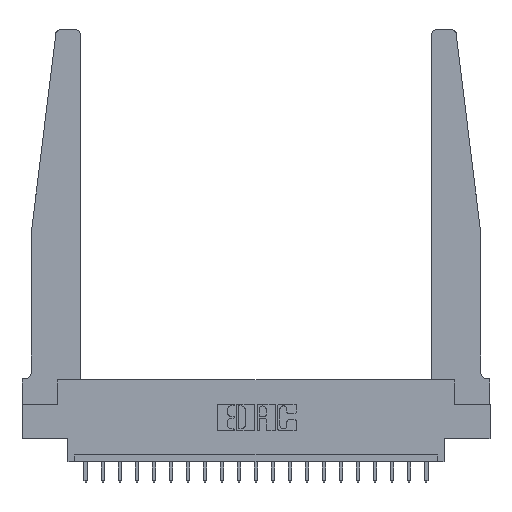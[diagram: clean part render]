
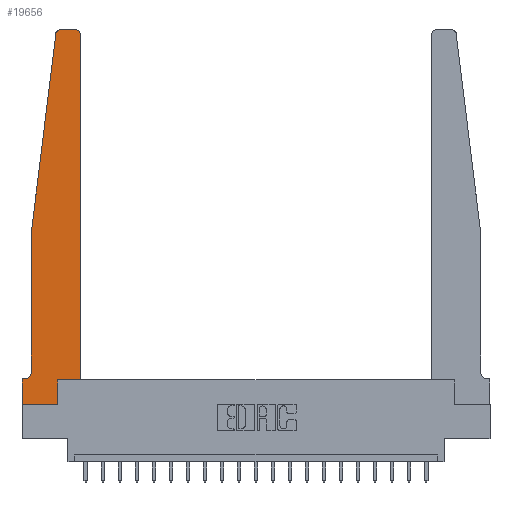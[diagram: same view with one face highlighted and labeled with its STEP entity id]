
A CAD part, top view. The second image highlights one B-rep face of the part: STEP entity #19656.
In plain terms, the highlighted planar face has unit normal (0, 0, 1).
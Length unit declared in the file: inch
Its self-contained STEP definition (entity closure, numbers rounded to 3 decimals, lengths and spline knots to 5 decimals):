
#21 = CARTESIAN_POINT ( 'NONE',  ( 0.065, 0.2375, 0.37 ) ) ;
#108 = VERTEX_POINT ( 'NONE', #7476 ) ;
#614 = LINE ( 'NONE', #13580, #15543 ) ;
#941 = DIRECTION ( 'NONE',  ( 1., 0., 0. ) ) ;
#1406 = EDGE_CURVE ( 'NONE', #4958, #7161, #15280, .T. ) ;
#1750 = CARTESIAN_POINT ( 'NONE',  ( 0.2605, 0.18, 0.37 ) ) ;
#2134 = ORIENTED_EDGE ( 'NONE', *, *, #15273, .T. ) ;
#2272 = ORIENTED_EDGE ( 'NONE', *, *, #1406, .T. ) ;
#2599 = DIRECTION ( 'NONE',  ( 0., 0., -1. ) ) ;
#2817 = ORIENTED_EDGE ( 'NONE', *, *, #3318, .T. ) ;
#3095 = ORIENTED_EDGE ( 'NONE', *, *, #17655, .T. ) ;
#3299 = ORIENTED_EDGE ( 'NONE', *, *, #13566, .T. ) ;
#3318 = EDGE_CURVE ( 'NONE', #15799, #108, #10245, .T. ) ;
#3681 = AXIS2_PLACEMENT_3D ( 'NONE', #21122, #14451, #14241 ) ;
#3939 = DIRECTION ( 'NONE',  ( 0., -1., 0. ) ) ;
#3965 = EDGE_CURVE ( 'NONE', #4890, #17208, #18164, .T. ) ;
#4087 = AXIS2_PLACEMENT_3D ( 'NONE', #6137, #8046, #15952 ) ;
#4551 = ORIENTED_EDGE ( 'NONE', *, *, #17848, .T. ) ;
#4890 = VERTEX_POINT ( 'NONE', #15218 ) ;
#4958 = VERTEX_POINT ( 'NONE', #20593 ) ;
#5138 = VECTOR ( 'NONE', #11738, 39.37008 ) ;
#5883 = CARTESIAN_POINT ( 'NONE',  ( 0.425, 0.18, 0.37 ) ) ;
#5889 = CARTESIAN_POINT ( 'NONE',  ( 0.425, 0.18, 0.37 ) ) ;
#6137 = CARTESIAN_POINT ( 'NONE',  ( 0.27653, 2.72, 0.37 ) ) ;
#6249 = CARTESIAN_POINT ( 'NONE',  ( 0.395, 2.72, 0.37 ) ) ;
#6349 = DIRECTION ( 'NONE',  ( 1., 0., 0. ) ) ;
#6737 = CARTESIAN_POINT ( 'NONE',  ( 0.065, 1.25, 0.37 ) ) ;
#6746 = EDGE_CURVE ( 'NONE', #108, #14042, #17950, .T. ) ;
#6750 = DIRECTION ( 'NONE',  ( -1., 0., 0. ) ) ;
#6759 = CIRCLE ( 'NONE', #9444, 0.05 ) ;
#7161 = VERTEX_POINT ( 'NONE', #1750 ) ;
#7476 = CARTESIAN_POINT ( 'NONE',  ( 0.24675, 2.72367, 0.37 ) ) ;
#7644 = LINE ( 'NONE', #12654, #20447 ) ;
#8046 = DIRECTION ( 'NONE',  ( 0., 0., 1. ) ) ;
#8259 = CARTESIAN_POINT ( 'NONE',  ( 0.25, 2.75, 0.37 ) ) ;
#8447 = VERTEX_POINT ( 'NONE', #5883 ) ;
#8603 = CARTESIAN_POINT ( 'NONE',  ( 0.425, 0.18, 0.37 ) ) ;
#8801 = LINE ( 'NONE', #8603, #10506 ) ;
#8855 = CARTESIAN_POINT ( 'NONE',  ( 0., 0., 0.37 ) ) ;
#9163 = VERTEX_POINT ( 'NONE', #12025 ) ;
#9293 = CARTESIAN_POINT ( 'NONE',  ( 0.065, 1.25, 0.37 ) ) ;
#9444 = AXIS2_PLACEMENT_3D ( 'NONE', #15856, #2599, #20381 ) ;
#9493 = CARTESIAN_POINT ( 'NONE',  ( 0.425, 2.72, 0.37 ) ) ;
#10059 = ORIENTED_EDGE ( 'NONE', *, *, #11629, .T. ) ;
#10174 = LINE ( 'NONE', #8259, #20086 ) ;
#10245 = CIRCLE ( 'NONE', #4087, 0.03 ) ;
#10506 = VECTOR ( 'NONE', #18427, 39.37008 ) ;
#10508 = AXIS2_PLACEMENT_3D ( 'NONE', #6249, #19416, #6349 ) ;
#11250 = PLANE ( 'NONE',  #3681 ) ;
#11629 = EDGE_CURVE ( 'NONE', #19287, #9163, #19748, .T. ) ;
#11723 = ORIENTED_EDGE ( 'NONE', *, *, #12429, .T. ) ;
#11738 = DIRECTION ( 'NONE',  ( -1., 0., 0. ) ) ;
#12025 = CARTESIAN_POINT ( 'NONE',  ( 0.395, 2.75, 0.37 ) ) ;
#12171 = DIRECTION ( 'NONE',  ( 0., -1., 0. ) ) ;
#12221 = EDGE_CURVE ( 'NONE', #9163, #15799, #10174, .T. ) ;
#12429 = EDGE_CURVE ( 'NONE', #14042, #12829, #614, .T. ) ;
#12654 = CARTESIAN_POINT ( 'NONE',  ( 0., 0., 0.37 ) ) ;
#12687 = CARTESIAN_POINT ( 'NONE',  ( 0., 0.1875, 0.37 ) ) ;
#12829 = VERTEX_POINT ( 'NONE', #21 ) ;
#13028 = VECTOR ( 'NONE', #19688, 39.37008 ) ;
#13553 = CARTESIAN_POINT ( 'NONE',  ( 0.065, 0.1875, 0.37 ) ) ;
#13566 = EDGE_CURVE ( 'NONE', #7161, #8447, #18729, .T. ) ;
#13580 = CARTESIAN_POINT ( 'NONE',  ( 0.065, 1.25, 0.37 ) ) ;
#13930 = VECTOR ( 'NONE', #19025, 39.37008 ) ;
#14042 = VERTEX_POINT ( 'NONE', #9293 ) ;
#14105 = EDGE_LOOP ( 'NONE', ( #16963, #2817, #19801, #11723, #20723, #18368, #2134, #3095, #2272, #3299, #4551, #10059 ) ) ;
#14202 = VECTOR ( 'NONE', #12171, 39.37008 ) ;
#14241 = DIRECTION ( 'NONE',  ( 1., 0., 0. ) ) ;
#14451 = DIRECTION ( 'NONE',  ( 0., 0., 1. ) ) ;
#15118 = VERTEX_POINT ( 'NONE', #8855 ) ;
#15218 = CARTESIAN_POINT ( 'NONE',  ( 0.015, 0.1875, 0.37 ) ) ;
#15273 = EDGE_CURVE ( 'NONE', #17208, #15118, #15393, .T. ) ;
#15280 = LINE ( 'NONE', #20218, #13930 ) ;
#15393 = LINE ( 'NONE', #20329, #14202 ) ;
#15543 = VECTOR ( 'NONE', #3939, 39.37008 ) ;
#15799 = VERTEX_POINT ( 'NONE', #20199 ) ;
#15856 = CARTESIAN_POINT ( 'NONE',  ( 0.015, 0.2375, 0.37 ) ) ;
#15952 = DIRECTION ( 'NONE',  ( 1., 0., 0. ) ) ;
#16963 = ORIENTED_EDGE ( 'NONE', *, *, #12221, .T. ) ;
#17208 = VERTEX_POINT ( 'NONE', #12687 ) ;
#17644 = EDGE_CURVE ( 'NONE', #12829, #4890, #6759, .T. ) ;
#17655 = EDGE_CURVE ( 'NONE', #15118, #4958, #7644, .T. ) ;
#17848 = EDGE_CURVE ( 'NONE', #8447, #19287, #8801, .T. ) ;
#17861 = FACE_OUTER_BOUND ( 'NONE', #14105, .T. ) ;
#17950 = LINE ( 'NONE', #6737, #13028 ) ;
#18164 = LINE ( 'NONE', #13553, #5138 ) ;
#18368 = ORIENTED_EDGE ( 'NONE', *, *, #3965, .T. ) ;
#18427 = DIRECTION ( 'NONE',  ( 0., 1., 0. ) ) ;
#18729 = LINE ( 'NONE', #5889, #20654 ) ;
#18879 = DIRECTION ( 'NONE',  ( 1., 0., 0. ) ) ;
#19025 = DIRECTION ( 'NONE',  ( 0., 1., 0. ) ) ;
#19287 = VERTEX_POINT ( 'NONE', #9493 ) ;
#19416 = DIRECTION ( 'NONE',  ( 0., 0., 1. ) ) ;
#19656 = ADVANCED_FACE ( 'NONE', ( #17861 ), #11250, .T. ) ;
#19688 = DIRECTION ( 'NONE',  ( -0.122, -0.992, 0. ) ) ;
#19748 = CIRCLE ( 'NONE', #10508, 0.03 ) ;
#19801 = ORIENTED_EDGE ( 'NONE', *, *, #6746, .T. ) ;
#20086 = VECTOR ( 'NONE', #6750, 39.37008 ) ;
#20199 = CARTESIAN_POINT ( 'NONE',  ( 0.27653, 2.75, 0.37 ) ) ;
#20218 = CARTESIAN_POINT ( 'NONE',  ( 0.2605, 0.18, 0.37 ) ) ;
#20329 = CARTESIAN_POINT ( 'NONE',  ( 0., 0., 0.37 ) ) ;
#20381 = DIRECTION ( 'NONE',  ( -1., 0., 0. ) ) ;
#20447 = VECTOR ( 'NONE', #18879, 39.37008 ) ;
#20593 = CARTESIAN_POINT ( 'NONE',  ( 0.2605, 0., 0.37 ) ) ;
#20654 = VECTOR ( 'NONE', #941, 39.37008 ) ;
#20723 = ORIENTED_EDGE ( 'NONE', *, *, #17644, .T. ) ;
#21122 = CARTESIAN_POINT ( 'NONE',  ( 0., 0.1875, 0.37 ) ) ;
